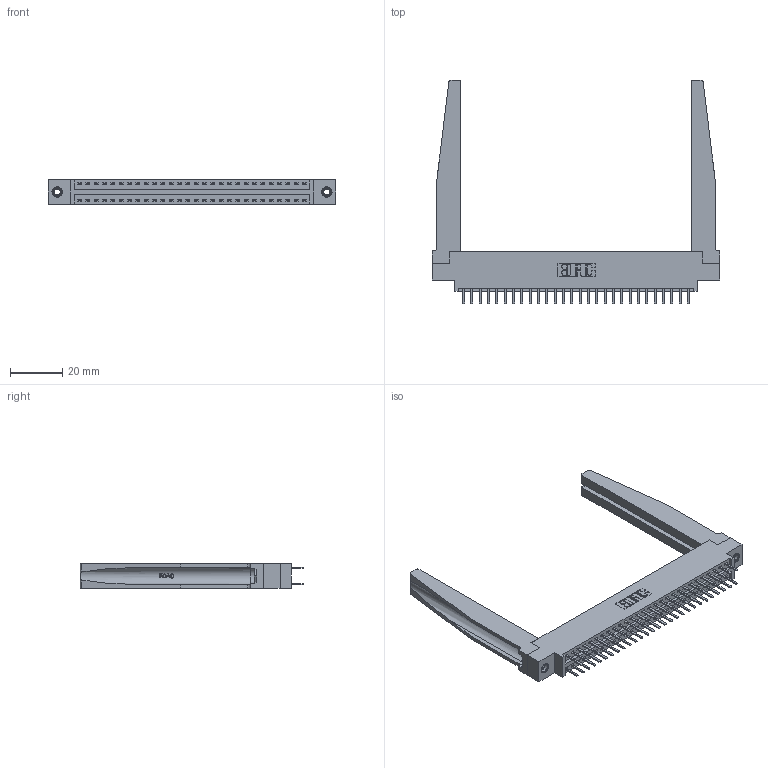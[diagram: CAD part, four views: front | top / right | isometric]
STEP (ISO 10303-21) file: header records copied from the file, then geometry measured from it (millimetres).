
FILE_DESCRIPTION (( 'STEP AP203' ), '1' );
FILE_NAME ('396-056-520-878.STEP', '2019-11-02T08:12:01', ( '' ), ( '' ), 'SwSTEP 2.0', 'SolidWorks 2016', '' );
FILE_SCHEMA (( 'CONFIG_CONTROL_DESIGN' ));
Length unit declared in the file: inch
Products named in the file (5): 346 Part_0.170 Offset - 0.156 Dia-TH; 345-292-001_345-293-120; 346-220-078_345-220-078; 345-250-001_345-250-001-102; 396-056-520-878
Assembly tree (61 placements, depth 2):
  396-056-520-878
    346 Part_0.170 Offset - 0.156 Dia-TH
    345-292-001_345-293-120  x56
    346-220-078_345-220-078  x2
    345-250-001_345-250-001-102  x2
Bounding box: 109.47 x 85.29 x 9.4 mm (x, y, z)
Volume: 17296 mm3; surface area: 20717.2 mm2
Topology: 61 solids, 61 shells, 3496 faces, 10077 edges, 6558 vertices
Faces by surface type: plane 2294, cylinder 1150, bspline 36, cone 12, torus 4
Entity records: 25152 total; most frequent: CARTESIAN_POINT 5115, ORIENTED_EDGE 3926, DIRECTION 3533, EDGE_CURVE 1963, VECTOR 1621, LINE 1621, VERTEX_POINT 1300, AXIS2_PLACEMENT_3D 956
